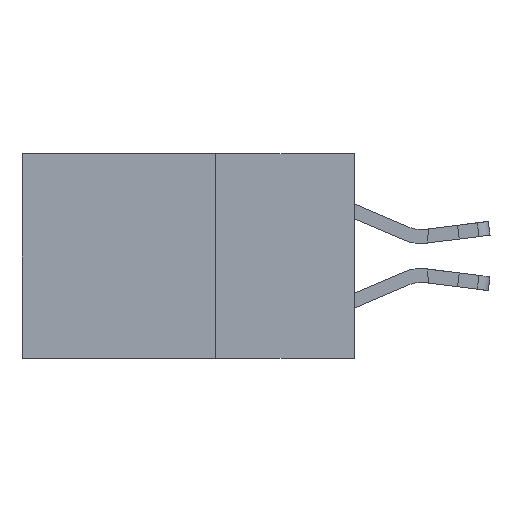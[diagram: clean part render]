
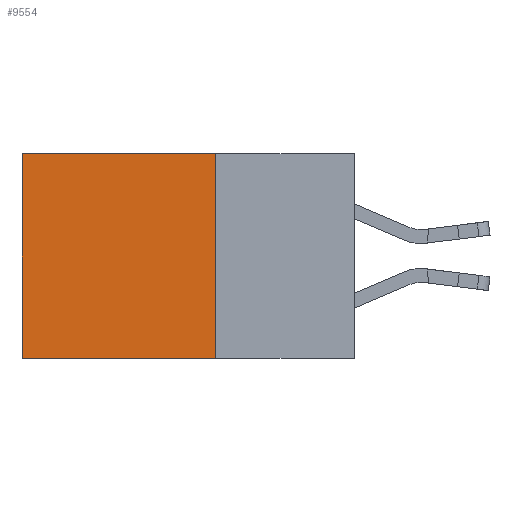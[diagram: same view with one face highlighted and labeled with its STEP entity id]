
A CAD part, left-side view. The second image highlights one B-rep face of the part: STEP entity #9554.
In plain terms, the highlighted planar face has unit normal (-1, 0, 0).
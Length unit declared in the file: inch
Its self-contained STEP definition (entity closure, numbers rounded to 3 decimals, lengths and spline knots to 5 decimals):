
#1 = DIRECTION ( 'NONE',  ( 0., 0., -1. ) ) ;
#170 = VECTOR ( 'NONE', #13287, 39.37008 ) ;
#1021 = PLANE ( 'NONE',  #2067 ) ;
#1058 = DIRECTION ( 'NONE',  ( 0., 1., 0. ) ) ;
#1217 = LINE ( 'NONE', #2058, #1453 ) ;
#1453 = VECTOR ( 'NONE', #1, 39.37008 ) ;
#2058 = CARTESIAN_POINT ( 'NONE',  ( 0.2615, 0.25, -0.37 ) ) ;
#2067 = AXIS2_PLACEMENT_3D ( 'NONE', #6731, #10844, #7665 ) ;
#2131 = ORIENTED_EDGE ( 'NONE', *, *, #3972, .F. ) ;
#2322 = EDGE_CURVE ( 'NONE', #9196, #4632, #9432, .T. ) ;
#2602 = CARTESIAN_POINT ( 'NONE',  ( 0.2615, 0.6, -0.37 ) ) ;
#2778 = VERTEX_POINT ( 'NONE', #5085 ) ;
#3377 = CARTESIAN_POINT ( 'NONE',  ( 0.2615, 0.25, -0.37 ) ) ;
#3972 = EDGE_CURVE ( 'NONE', #11770, #4632, #5742, .T. ) ;
#4365 = FACE_OUTER_BOUND ( 'NONE', #7577, .T. ) ;
#4619 = EDGE_CURVE ( 'NONE', #2778, #9196, #6343, .T. ) ;
#4632 = VERTEX_POINT ( 'NONE', #13105 ) ;
#4665 = ORIENTED_EDGE ( 'NONE', *, *, #2322, .T. ) ;
#5085 = CARTESIAN_POINT ( 'NONE',  ( 0.2615, 0.25, 0. ) ) ;
#5349 = ORIENTED_EDGE ( 'NONE', *, *, #4619, .T. ) ;
#5742 = LINE ( 'NONE', #3377, #170 ) ;
#5810 = CARTESIAN_POINT ( 'NONE',  ( 0.2615, 0.6, 0. ) ) ;
#6343 = LINE ( 'NONE', #12890, #7019 ) ;
#6731 = CARTESIAN_POINT ( 'NONE',  ( 0.2615, 0.25, -0.37 ) ) ;
#7019 = VECTOR ( 'NONE', #1058, 39.37008 ) ;
#7577 = EDGE_LOOP ( 'NONE', ( #4665, #2131, #8518, #5349 ) ) ;
#7665 = DIRECTION ( 'NONE',  ( 0., 0., -1. ) ) ;
#8279 = CARTESIAN_POINT ( 'NONE',  ( 0.2615, 0.25, -0.37 ) ) ;
#8518 = ORIENTED_EDGE ( 'NONE', *, *, #13851, .F. ) ;
#9196 = VERTEX_POINT ( 'NONE', #5810 ) ;
#9357 = DIRECTION ( 'NONE',  ( 0., 0., -1. ) ) ;
#9432 = LINE ( 'NONE', #2602, #13646 ) ;
#9554 = ADVANCED_FACE ( 'NONE', ( #4365 ), #1021, .F. ) ;
#10844 = DIRECTION ( 'NONE',  ( 1., 0., 0. ) ) ;
#11770 = VERTEX_POINT ( 'NONE', #8279 ) ;
#12890 = CARTESIAN_POINT ( 'NONE',  ( 0.2615, 0.25, 0. ) ) ;
#13105 = CARTESIAN_POINT ( 'NONE',  ( 0.2615, 0.6, -0.37 ) ) ;
#13287 = DIRECTION ( 'NONE',  ( 0., 1., 0. ) ) ;
#13646 = VECTOR ( 'NONE', #9357, 39.37008 ) ;
#13851 = EDGE_CURVE ( 'NONE', #2778, #11770, #1217, .T. ) ;
